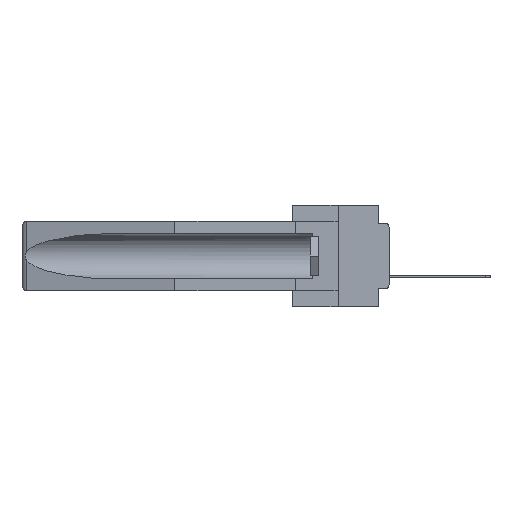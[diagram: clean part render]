
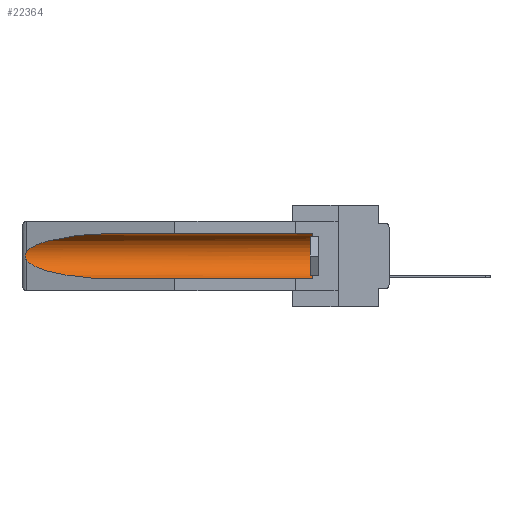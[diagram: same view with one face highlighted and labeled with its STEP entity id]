
A CAD part, left-side view. The second image highlights one B-rep face of the part: STEP entity #22364.
In plain terms, the highlighted cylindrical face has radius 2.857 mm (diameter 5.715 mm), a partial arc.
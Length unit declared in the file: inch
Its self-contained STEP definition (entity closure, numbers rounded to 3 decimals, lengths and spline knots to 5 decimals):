
#23 = CARTESIAN_POINT ( 'NONE',  ( 0.2675, 1.53308, -0.17534 ) ) ;
#123 = CARTESIAN_POINT ( 'NONE',  ( 0.155, 1.07973, -0.059 ) ) ;
#386 = AXIS2_PLACEMENT_3D ( 'NONE', #13205, #13659, #31619 ) ;
#1884 = B_SPLINE_CURVE_WITH_KNOTS ( 'NONE', 3,
 ( #32922, #22904, #20291, #7553, #25490, #23, #5173, #20176, #7777, #33275 ),
 .UNSPECIFIED., .F., .F.,
 ( 4, 2, 2, 2, 4 ),
 ( 0., 0.00029, 0.00058, 0.00087, 0.00117 ),
 .UNSPECIFIED. ) ;
#2288 = VERTEX_POINT ( 'NONE', #2647 ) ;
#2428 = CARTESIAN_POINT ( 'NONE',  ( 0.155, -0.30754, -0.059 ) ) ;
#2647 = CARTESIAN_POINT ( 'NONE',  ( 0.155, 1.07973, -0.284 ) ) ;
#2941 = EDGE_CURVE ( 'NONE', #24581, #2288, #16267, .T. ) ;
#3160 = CARTESIAN_POINT ( 'NONE',  ( 0.155, 1.07973, -0.059 ) ) ;
#3882 = DIRECTION ( 'NONE',  ( 0., 1., 0. ) ) ;
#4138 = ORIENTED_EDGE ( 'NONE', *, *, #29864, .T. ) ;
#4340 = VECTOR ( 'NONE', #3882, 39.37008 ) ;
#4569 = LINE ( 'NONE', #2428, #22612 ) ;
#5173 = CARTESIAN_POINT ( 'NONE',  ( 0.2673, 1.53269, -0.17917 ) ) ;
#5350 = DIRECTION ( 'NONE',  ( 0., 1., 0. ) ) ;
#5554 = AXIS2_PLACEMENT_3D ( 'NONE', #20948, #28988, #26264 ) ;
#5741 = CARTESIAN_POINT ( 'NONE',  ( 0.25451, 1.48313, -0.09465 ) ) ;
#6142 = ORIENTED_EDGE ( 'NONE', *, *, #2941, .T. ) ;
#7148 = LINE ( 'NONE', #19204, #4340 ) ;
#7553 = CARTESIAN_POINT ( 'NONE',  ( 0.2673, 1.5327, -0.16383 ) ) ;
#7723 = EDGE_CURVE ( 'NONE', #15578, #11630, #15283, .T. ) ;
#7777 = CARTESIAN_POINT ( 'NONE',  ( 0.26597, 1.5296, -0.19026 ) ) ;
#10309 = EDGE_LOOP ( 'NONE', ( #23062, #12810, #6142, #11816, #16580, #4138 ) ) ;
#11222 = CIRCLE ( 'NONE', #5554, 0.1125 ) ;
#11630 = VERTEX_POINT ( 'NONE', #29294 ) ;
#11816 = ORIENTED_EDGE ( 'NONE', *, *, #14591, .F. ) ;
#11923 = FACE_OUTER_BOUND ( 'NONE', #10309, .T. ) ;
#12810 = ORIENTED_EDGE ( 'NONE', *, *, #23342, .T. ) ;
#13205 = CARTESIAN_POINT ( 'NONE',  ( 0.155, -0.30754, -0.1715 ) ) ;
#13468 = CARTESIAN_POINT ( 'NONE',  ( 0.25451, 1.48313, -0.24835 ) ) ;
#13659 = DIRECTION ( 'NONE',  ( 0., 1., 0. ) ) ;
#13722 = CARTESIAN_POINT ( 'NONE',  ( 0.26537, 1.52718, -0.14972 ) ) ;
#13946 = CARTESIAN_POINT ( 'NONE',  ( 0.21114, 1.30732, -0.059 ) ) ;
#14591 = EDGE_CURVE ( 'NONE', #29380, #2288, #7148, .T. ) ;
#15283 =( BOUNDED_CURVE ( )  B_SPLINE_CURVE ( 3, ( #3160, #13946, #5741, #13722 ),
 .UNSPECIFIED., .F., .F. ) 
 B_SPLINE_CURVE_WITH_KNOTS ( ( 4, 4 ),
 ( 4.71239, 6.08839 ),
 .UNSPECIFIED. ) 
 CURVE ( )  GEOMETRIC_REPRESENTATION_ITEM ( )  RATIONAL_B_SPLINE_CURVE ( ( 1., 0.848, 0.848, 1. ) ) 
 REPRESENTATION_ITEM ( '' )  );
#15578 = VERTEX_POINT ( 'NONE', #123 ) ;
#15717 = CARTESIAN_POINT ( 'NONE',  ( 0.21114, 1.30732, -0.284 ) ) ;
#16267 =( BOUNDED_CURVE ( )  B_SPLINE_CURVE ( 3, ( #31112, #13468, #15717, #21049 ),
 .UNSPECIFIED., .F., .F. ) 
 B_SPLINE_CURVE_WITH_KNOTS ( ( 4, 4 ),
 ( 0.1948, 1.5708 ),
 .UNSPECIFIED. ) 
 CURVE ( )  GEOMETRIC_REPRESENTATION_ITEM ( )  RATIONAL_B_SPLINE_CURVE ( ( 1., 0.848, 0.848, 1. ) ) 
 REPRESENTATION_ITEM ( '' )  );
#16580 = ORIENTED_EDGE ( 'NONE', *, *, #20401, .T. ) ;
#19204 = CARTESIAN_POINT ( 'NONE',  ( 0.155, -0.30754, -0.284 ) ) ;
#20176 = CARTESIAN_POINT ( 'NONE',  ( 0.26655, 1.53094, -0.18657 ) ) ;
#20291 = CARTESIAN_POINT ( 'NONE',  ( 0.26654, 1.53092, -0.15636 ) ) ;
#20401 = EDGE_CURVE ( 'NONE', #29380, #24994, #11222, .T. ) ;
#20948 = CARTESIAN_POINT ( 'NONE',  ( 0.155, 0.126, -0.1715 ) ) ;
#21049 = CARTESIAN_POINT ( 'NONE',  ( 0.155, 1.07973, -0.284 ) ) ;
#21445 = CYLINDRICAL_SURFACE ( 'NONE', #386, 0.1125 ) ;
#21576 = CARTESIAN_POINT ( 'NONE',  ( 0.155, 0.126, -0.284 ) ) ;
#22364 = ADVANCED_FACE ( 'NONE', ( #11923 ), #21445, .F. ) ;
#22596 = CARTESIAN_POINT ( 'NONE',  ( 0.26537, 1.52718, -0.19328 ) ) ;
#22612 = VECTOR ( 'NONE', #5350, 39.37008 ) ;
#22904 = CARTESIAN_POINT ( 'NONE',  ( 0.26597, 1.52961, -0.15275 ) ) ;
#23062 = ORIENTED_EDGE ( 'NONE', *, *, #7723, .T. ) ;
#23342 = EDGE_CURVE ( 'NONE', #11630, #24581, #1884, .T. ) ;
#24581 = VERTEX_POINT ( 'NONE', #22596 ) ;
#24994 = VERTEX_POINT ( 'NONE', #32871 ) ;
#25490 = CARTESIAN_POINT ( 'NONE',  ( 0.2675, 1.53308, -0.16763 ) ) ;
#26264 = DIRECTION ( 'NONE',  ( 0., 0., 1. ) ) ;
#28988 = DIRECTION ( 'NONE',  ( 0., -1., 0. ) ) ;
#29294 = CARTESIAN_POINT ( 'NONE',  ( 0.26537, 1.52718, -0.14972 ) ) ;
#29380 = VERTEX_POINT ( 'NONE', #21576 ) ;
#29864 = EDGE_CURVE ( 'NONE', #24994, #15578, #4569, .T. ) ;
#31112 = CARTESIAN_POINT ( 'NONE',  ( 0.26537, 1.52718, -0.19328 ) ) ;
#31619 = DIRECTION ( 'NONE',  ( 0., 0., 1. ) ) ;
#32871 = CARTESIAN_POINT ( 'NONE',  ( 0.155, 0.126, -0.059 ) ) ;
#32922 = CARTESIAN_POINT ( 'NONE',  ( 0.26537, 1.52718, -0.14972 ) ) ;
#33275 = CARTESIAN_POINT ( 'NONE',  ( 0.26537, 1.52718, -0.19328 ) ) ;
